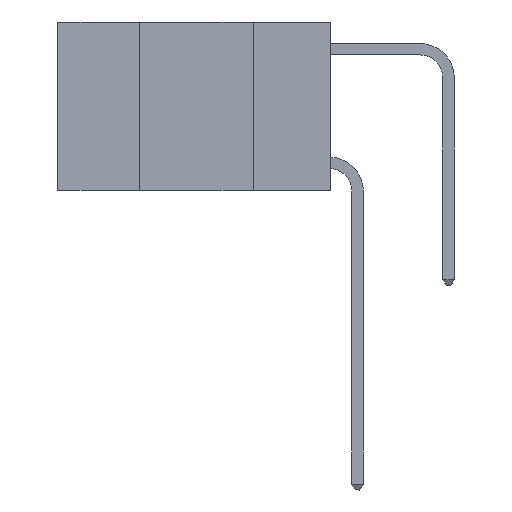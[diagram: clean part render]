
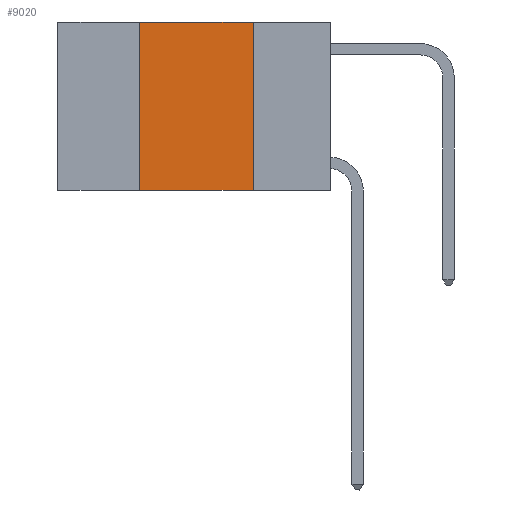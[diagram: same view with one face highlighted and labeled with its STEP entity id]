
A CAD part, left-side view. The second image highlights one B-rep face of the part: STEP entity #9020.
In plain terms, the highlighted planar face has unit normal (-1, 0, 0).
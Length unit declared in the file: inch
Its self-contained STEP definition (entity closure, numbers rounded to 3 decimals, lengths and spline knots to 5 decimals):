
#1070 = AXIS2_PLACEMENT_3D ( 'NONE', #2991, #13361, #5704 ) ;
#2843 = EDGE_CURVE ( 'NONE', #9654, #16110, #6836, .T. ) ;
#2991 = CARTESIAN_POINT ( 'NONE',  ( 0., 0.6, 0. ) ) ;
#3462 = LINE ( 'NONE', #8509, #16304 ) ;
#3523 = VERTEX_POINT ( 'NONE', #13297 ) ;
#3666 = EDGE_CURVE ( 'NONE', #16110, #3523, #3462, .T. ) ;
#4338 = PLANE ( 'NONE',  #1070 ) ;
#4498 = VECTOR ( 'NONE', #11264, 39.37008 ) ;
#4551 = EDGE_CURVE ( 'NONE', #12600, #9654, #8003, .T. ) ;
#4809 = VECTOR ( 'NONE', #10569, 39.37008 ) ;
#4839 = CARTESIAN_POINT ( 'NONE',  ( 0., 0.42, -0.37 ) ) ;
#5704 = DIRECTION ( 'NONE',  ( 0., 0., -1. ) ) ;
#6836 = LINE ( 'NONE', #12821, #16536 ) ;
#7244 = DIRECTION ( 'NONE',  ( 0., 0., -1. ) ) ;
#7387 = CARTESIAN_POINT ( 'NONE',  ( 0., 0.42, 0. ) ) ;
#7826 = ORIENTED_EDGE ( 'NONE', *, *, #3666, .F. ) ;
#8003 = LINE ( 'NONE', #7387, #4498 ) ;
#8079 = EDGE_CURVE ( 'NONE', #12600, #3523, #15054, .T. ) ;
#8250 = ORIENTED_EDGE ( 'NONE', *, *, #2843, .F. ) ;
#8395 = ORIENTED_EDGE ( 'NONE', *, *, #4551, .F. ) ;
#8400 = CARTESIAN_POINT ( 'NONE',  ( 0., 0.42, 0. ) ) ;
#8465 = ORIENTED_EDGE ( 'NONE', *, *, #8079, .T. ) ;
#8509 = CARTESIAN_POINT ( 'NONE',  ( 0., 0.17, 0. ) ) ;
#9020 = ADVANCED_FACE ( 'NONE', ( #9884 ), #4338, .F. ) ;
#9314 = CARTESIAN_POINT ( 'NONE',  ( 0., 0.6, -0.37 ) ) ;
#9654 = VERTEX_POINT ( 'NONE', #8400 ) ;
#9884 = FACE_OUTER_BOUND ( 'NONE', #13189, .T. ) ;
#10569 = DIRECTION ( 'NONE',  ( 0., -1., 0. ) ) ;
#11264 = DIRECTION ( 'NONE',  ( 0., 0., 1. ) ) ;
#12600 = VERTEX_POINT ( 'NONE', #4839 ) ;
#12821 = CARTESIAN_POINT ( 'NONE',  ( 0., 0.6, 0. ) ) ;
#13189 = EDGE_LOOP ( 'NONE', ( #7826, #8250, #8395, #8465 ) ) ;
#13297 = CARTESIAN_POINT ( 'NONE',  ( 0., 0.17, -0.37 ) ) ;
#13361 = DIRECTION ( 'NONE',  ( 1., 0., 0. ) ) ;
#14079 = DIRECTION ( 'NONE',  ( 0., -1., 0. ) ) ;
#14496 = CARTESIAN_POINT ( 'NONE',  ( 0., 0.17, 0. ) ) ;
#15054 = LINE ( 'NONE', #9314, #4809 ) ;
#16110 = VERTEX_POINT ( 'NONE', #14496 ) ;
#16304 = VECTOR ( 'NONE', #7244, 39.37008 ) ;
#16536 = VECTOR ( 'NONE', #14079, 39.37008 ) ;
